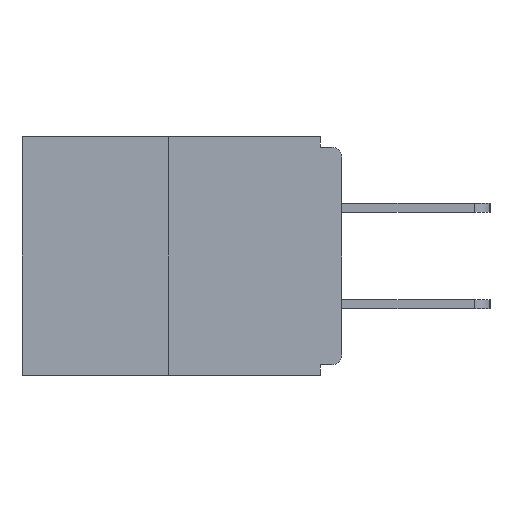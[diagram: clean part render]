
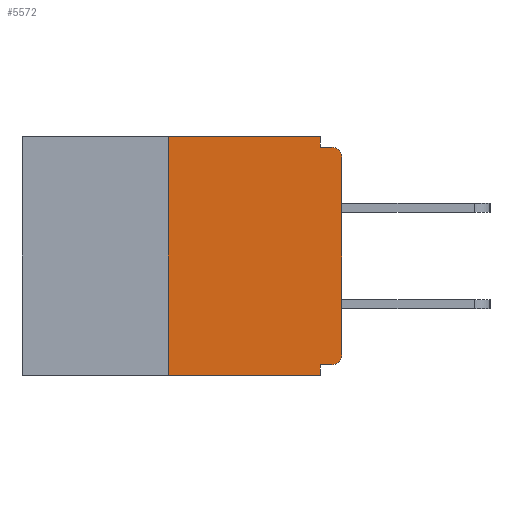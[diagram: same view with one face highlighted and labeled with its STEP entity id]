
A CAD part, left-side view. The second image highlights one B-rep face of the part: STEP entity #5572.
In plain terms, the highlighted planar face has unit normal (-1, 0, 0).
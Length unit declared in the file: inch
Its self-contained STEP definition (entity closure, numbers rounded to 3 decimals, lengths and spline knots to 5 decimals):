
#781 = LINE ( 'NONE', #13709, #13100 ) ;
#876 = PLANE ( 'NONE',  #12430 ) ;
#1220 = VECTOR ( 'NONE', #19004, 39.37008 ) ;
#1474 = EDGE_CURVE ( 'NONE', #9772, #6661, #5310, .T. ) ;
#1501 = CARTESIAN_POINT ( 'NONE',  ( 0., 0., -0.313 ) ) ;
#1544 = DIRECTION ( 'NONE',  ( 0., -1., 0. ) ) ;
#1645 = ORIENTED_EDGE ( 'NONE', *, *, #8129, .T. ) ;
#1942 = EDGE_CURVE ( 'NONE', #10596, #3939, #9062, .T. ) ;
#1985 = DIRECTION ( 'NONE',  ( 0., 0., 1. ) ) ;
#1986 = ORIENTED_EDGE ( 'NONE', *, *, #1942, .T. ) ;
#2049 = ORIENTED_EDGE ( 'NONE', *, *, #14293, .T. ) ;
#2255 = EDGE_CURVE ( 'NONE', #6661, #3939, #18062, .T. ) ;
#2439 = CARTESIAN_POINT ( 'NONE',  ( 0., 0.031, 0. ) ) ;
#2744 = CARTESIAN_POINT ( 'NONE',  ( 0., 0.25, 0. ) ) ;
#3005 = CARTESIAN_POINT ( 'NONE',  ( 0., 0.031, -0.343 ) ) ;
#3303 = CARTESIAN_POINT ( 'NONE',  ( 0., 0., -0.328 ) ) ;
#3327 = EDGE_CURVE ( 'NONE', #18183, #9772, #18026, .T. ) ;
#3939 = VERTEX_POINT ( 'NONE', #17050 ) ;
#3959 = VERTEX_POINT ( 'NONE', #3005 ) ;
#4245 = VERTEX_POINT ( 'NONE', #7482 ) ;
#4302 = CARTESIAN_POINT ( 'NONE',  ( 0., 0.031, 0. ) ) ;
#4666 = CARTESIAN_POINT ( 'NONE',  ( 0., 0., 0. ) ) ;
#5310 = LINE ( 'NONE', #4302, #12147 ) ;
#5572 = ADVANCED_FACE ( 'NONE', ( #17431 ), #876, .F. ) ;
#5669 = DIRECTION ( 'NONE',  ( 0., 1., 0. ) ) ;
#5674 = VERTEX_POINT ( 'NONE', #1501 ) ;
#5812 = DIRECTION ( 'NONE',  ( -1., 0., 0. ) ) ;
#5952 = CARTESIAN_POINT ( 'NONE',  ( 0., 0.015, -0.313 ) ) ;
#6159 = AXIS2_PLACEMENT_3D ( 'NONE', #16695, #11983, #13563 ) ;
#6561 = ORIENTED_EDGE ( 'NONE', *, *, #1474, .F. ) ;
#6661 = VERTEX_POINT ( 'NONE', #13951 ) ;
#6821 = VECTOR ( 'NONE', #17458, 39.37008 ) ;
#7107 = DIRECTION ( 'NONE',  ( 0., 0., -1. ) ) ;
#7482 = CARTESIAN_POINT ( 'NONE',  ( 0., 0.031, -0.328 ) ) ;
#7528 = LINE ( 'NONE', #18257, #15022 ) ;
#7682 = DIRECTION ( 'NONE',  ( 0., 0., -1. ) ) ;
#8047 = EDGE_CURVE ( 'NONE', #9109, #5674, #16351, .T. ) ;
#8129 = EDGE_CURVE ( 'NONE', #5674, #10596, #11134, .T. ) ;
#9062 = CIRCLE ( 'NONE', #6159, 0.015 ) ;
#9109 = VERTEX_POINT ( 'NONE', #11729 ) ;
#9490 = DIRECTION ( 'NONE',  ( 0., 0., 1. ) ) ;
#9772 = VERTEX_POINT ( 'NONE', #2439 ) ;
#10168 = EDGE_CURVE ( 'NONE', #18982, #18183, #7528, .T. ) ;
#10596 = VERTEX_POINT ( 'NONE', #13211 ) ;
#10629 = LINE ( 'NONE', #14067, #6821 ) ;
#10834 = VECTOR ( 'NONE', #1544, 39.37008 ) ;
#11134 = LINE ( 'NONE', #4666, #17133 ) ;
#11228 = CARTESIAN_POINT ( 'NONE',  ( 0., 0.25, -0.343 ) ) ;
#11729 = CARTESIAN_POINT ( 'NONE',  ( 0., 0.015, -0.328 ) ) ;
#11983 = DIRECTION ( 'NONE',  ( -1., 0., 0. ) ) ;
#12147 = VECTOR ( 'NONE', #7682, 39.37008 ) ;
#12430 = AXIS2_PLACEMENT_3D ( 'NONE', #18540, #13741, #16947 ) ;
#12527 = ORIENTED_EDGE ( 'NONE', *, *, #3327, .F. ) ;
#13028 = EDGE_LOOP ( 'NONE', ( #12527, #16532, #2049, #17457, #13441, #15799, #1645, #1986, #20313, #6561 ) ) ;
#13100 = VECTOR ( 'NONE', #7107, 39.37008 ) ;
#13211 = CARTESIAN_POINT ( 'NONE',  ( 0., 0., -0.03 ) ) ;
#13441 = ORIENTED_EDGE ( 'NONE', *, *, #14226, .F. ) ;
#13563 = DIRECTION ( 'NONE',  ( 0., 0., -1. ) ) ;
#13709 = CARTESIAN_POINT ( 'NONE',  ( 0., 0.031, -0.343 ) ) ;
#13741 = DIRECTION ( 'NONE',  ( 1., 0., 0. ) ) ;
#13951 = CARTESIAN_POINT ( 'NONE',  ( 0., 0.031, -0.015 ) ) ;
#14067 = CARTESIAN_POINT ( 'NONE',  ( 0., 0.46, -0.343 ) ) ;
#14226 = EDGE_CURVE ( 'NONE', #9109, #4245, #19608, .T. ) ;
#14293 = EDGE_CURVE ( 'NONE', #18982, #3959, #10629, .T. ) ;
#14344 = CARTESIAN_POINT ( 'NONE',  ( 0., 0., -0.015 ) ) ;
#14645 = EDGE_CURVE ( 'NONE', #4245, #3959, #781, .T. ) ;
#15022 = VECTOR ( 'NONE', #1985, 39.37008 ) ;
#15799 = ORIENTED_EDGE ( 'NONE', *, *, #8047, .T. ) ;
#16351 = CIRCLE ( 'NONE', #17403, 0.015 ) ;
#16532 = ORIENTED_EDGE ( 'NONE', *, *, #10168, .F. ) ;
#16695 = CARTESIAN_POINT ( 'NONE',  ( 0., 0.015, -0.03 ) ) ;
#16947 = DIRECTION ( 'NONE',  ( 0., 0., -1. ) ) ;
#17050 = CARTESIAN_POINT ( 'NONE',  ( 0., 0.015, -0.015 ) ) ;
#17133 = VECTOR ( 'NONE', #9490, 39.37008 ) ;
#17403 = AXIS2_PLACEMENT_3D ( 'NONE', #5952, #5812, #18914 ) ;
#17431 = FACE_OUTER_BOUND ( 'NONE', #13028, .T. ) ;
#17457 = ORIENTED_EDGE ( 'NONE', *, *, #14645, .F. ) ;
#17458 = DIRECTION ( 'NONE',  ( 0., -1., 0. ) ) ;
#18026 = LINE ( 'NONE', #19212, #1220 ) ;
#18062 = LINE ( 'NONE', #14344, #10834 ) ;
#18183 = VERTEX_POINT ( 'NONE', #2744 ) ;
#18257 = CARTESIAN_POINT ( 'NONE',  ( 0., 0.25, 0. ) ) ;
#18540 = CARTESIAN_POINT ( 'NONE',  ( 0., 0.46, 0. ) ) ;
#18914 = DIRECTION ( 'NONE',  ( 0., 0., -1. ) ) ;
#18982 = VERTEX_POINT ( 'NONE', #11228 ) ;
#19004 = DIRECTION ( 'NONE',  ( 0., -1., 0. ) ) ;
#19212 = CARTESIAN_POINT ( 'NONE',  ( 0., 0.46, 0. ) ) ;
#19608 = LINE ( 'NONE', #3303, #20133 ) ;
#20133 = VECTOR ( 'NONE', #5669, 39.37008 ) ;
#20313 = ORIENTED_EDGE ( 'NONE', *, *, #2255, .F. ) ;
